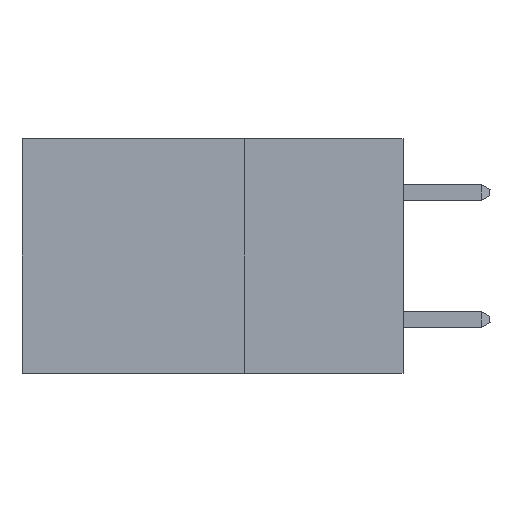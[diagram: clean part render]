
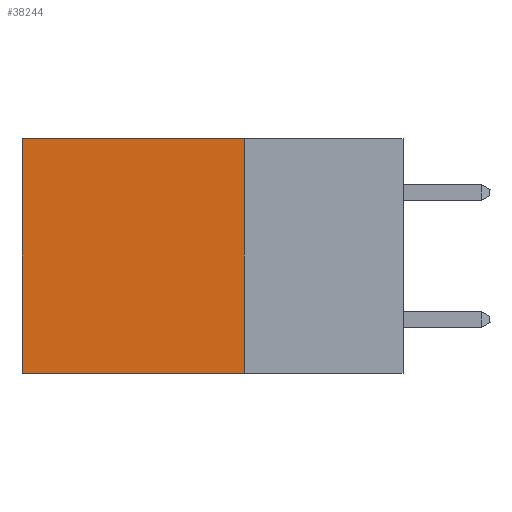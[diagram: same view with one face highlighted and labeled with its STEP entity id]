
A CAD part, left-side view. The second image highlights one B-rep face of the part: STEP entity #38244.
In plain terms, the highlighted planar face has unit normal (-1, 0, 0).
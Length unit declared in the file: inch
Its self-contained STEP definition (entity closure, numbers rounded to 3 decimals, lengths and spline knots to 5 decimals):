
#417 = EDGE_CURVE ( 'NONE', #10530, #8122, #12452, .T. ) ;
#5362 = ORIENTED_EDGE ( 'NONE', *, *, #39974, .F. ) ;
#6086 = DIRECTION ( 'NONE',  ( 0., 0., -1. ) ) ;
#6330 = LINE ( 'NONE', #12561, #17479 ) ;
#7350 = ORIENTED_EDGE ( 'NONE', *, *, #31045, .T. ) ;
#7355 = VERTEX_POINT ( 'NONE', #36493 ) ;
#8122 = VERTEX_POINT ( 'NONE', #15296 ) ;
#10530 = VERTEX_POINT ( 'NONE', #25305 ) ;
#11491 = VECTOR ( 'NONE', #21528, 39.37008 ) ;
#12146 = AXIS2_PLACEMENT_3D ( 'NONE', #12844, #28146, #22022 ) ;
#12244 = ORIENTED_EDGE ( 'NONE', *, *, #417, .F. ) ;
#12452 = LINE ( 'NONE', #28050, #11491 ) ;
#12561 = CARTESIAN_POINT ( 'NONE',  ( 0.2875, 0.6, 0. ) ) ;
#12609 = VECTOR ( 'NONE', #20437, 39.37008 ) ;
#12844 = CARTESIAN_POINT ( 'NONE',  ( 0.2875, 0.25, 0. ) ) ;
#15296 = CARTESIAN_POINT ( 'NONE',  ( 0.2875, 0.6, -0.37 ) ) ;
#17479 = VECTOR ( 'NONE', #6086, 39.37008 ) ;
#20314 = CARTESIAN_POINT ( 'NONE',  ( 0.2875, 0.25, 0. ) ) ;
#20437 = DIRECTION ( 'NONE',  ( 0., 0., -1. ) ) ;
#20894 = LINE ( 'NONE', #20314, #28168 ) ;
#21528 = DIRECTION ( 'NONE',  ( 0., 1., 0. ) ) ;
#22022 = DIRECTION ( 'NONE',  ( 0., 0., -1. ) ) ;
#25305 = CARTESIAN_POINT ( 'NONE',  ( 0.2875, 0.25, -0.37 ) ) ;
#26426 = DIRECTION ( 'NONE',  ( 0., 1., 0. ) ) ;
#27490 = EDGE_LOOP ( 'NONE', ( #7350, #12244, #5362, #29789 ) ) ;
#28050 = CARTESIAN_POINT ( 'NONE',  ( 0.2875, 0.25, -0.37 ) ) ;
#28146 = DIRECTION ( 'NONE',  ( 1., 0., 0. ) ) ;
#28168 = VECTOR ( 'NONE', #26426, 39.37008 ) ;
#29789 = ORIENTED_EDGE ( 'NONE', *, *, #30810, .T. ) ;
#30810 = EDGE_CURVE ( 'NONE', #36034, #7355, #20894, .T. ) ;
#31045 = EDGE_CURVE ( 'NONE', #7355, #8122, #6330, .T. ) ;
#35669 = FACE_OUTER_BOUND ( 'NONE', #27490, .T. ) ;
#35999 = CARTESIAN_POINT ( 'NONE',  ( 0.2875, 0.25, 0. ) ) ;
#36034 = VERTEX_POINT ( 'NONE', #35999 ) ;
#36493 = CARTESIAN_POINT ( 'NONE',  ( 0.2875, 0.6, 0. ) ) ;
#36932 = LINE ( 'NONE', #39100, #12609 ) ;
#37455 = PLANE ( 'NONE',  #12146 ) ;
#38244 = ADVANCED_FACE ( 'NONE', ( #35669 ), #37455, .F. ) ;
#39100 = CARTESIAN_POINT ( 'NONE',  ( 0.2875, 0.25, 0. ) ) ;
#39974 = EDGE_CURVE ( 'NONE', #36034, #10530, #36932, .T. ) ;
